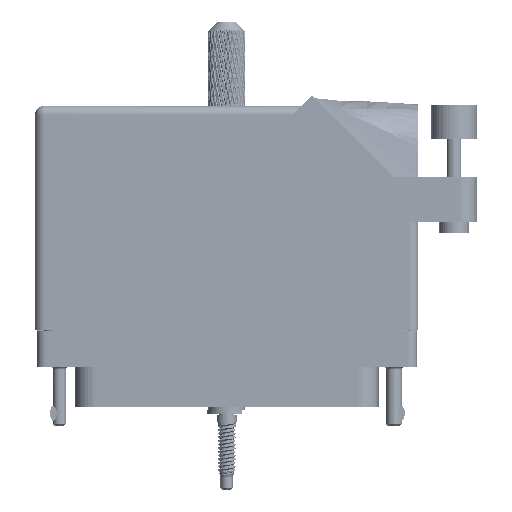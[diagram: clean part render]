
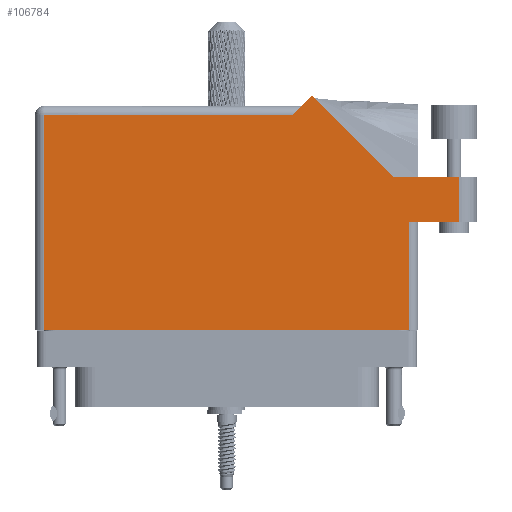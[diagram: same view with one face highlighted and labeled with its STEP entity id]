
A CAD part, front view. The second image highlights one B-rep face of the part: STEP entity #106784.
In plain terms, the highlighted face is planar.
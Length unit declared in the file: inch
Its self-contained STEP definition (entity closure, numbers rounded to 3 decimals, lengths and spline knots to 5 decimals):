
#1257 = CARTESIAN_POINT ( 'NONE',  ( 1.14042, 0.944, 0.455 ) ) ;
#1765 = ORIENTED_EDGE ( 'NONE', *, *, #94128, .T. ) ;
#3207 = ORIENTED_EDGE ( 'NONE', *, *, #35768, .T. ) ;
#3208 = ORIENTED_EDGE ( 'NONE', *, *, #44661, .T. ) ;
#7178 = CARTESIAN_POINT ( 'NONE',  ( -1.244, -0.1, 0.455 ) ) ;
#8013 = CARTESIAN_POINT ( 'NONE',  ( 1.244, 0.637, 0.455 ) ) ;
#8745 = ORIENTED_EDGE ( 'NONE', *, *, #76521, .T. ) ;
#10144 = VECTOR ( 'NONE', #37858, 39.37008 ) ;
#10283 = VERTEX_POINT ( 'NONE', #1257 ) ;
#11735 = EDGE_CURVE ( 'NONE', #63061, #35905, #89748, .T. ) ;
#12236 = DIRECTION ( 'NONE',  ( -0.707, -0.707, 0. ) ) ;
#13209 = LINE ( 'NONE', #78393, #10144 ) ;
#14014 = LINE ( 'NONE', #91039, #70665 ) ;
#14798 = DIRECTION ( 'NONE',  ( 0., -1., 0. ) ) ;
#16679 = PLANE ( 'NONE',  #77204 ) ;
#19233 = EDGE_CURVE ( 'NONE', #10283, #108725, #124353, .T. ) ;
#20253 = ORIENTED_EDGE ( 'NONE', *, *, #19233, .T. ) ;
#20635 = EDGE_CURVE ( 'NONE', #93317, #43607, #14014, .T. ) ;
#20872 = CARTESIAN_POINT ( 'NONE',  ( 0.451, 1.368, 0.455 ) ) ;
#24332 = VECTOR ( 'NONE', #41796, 39.37008 ) ;
#27872 = DIRECTION ( 'NONE',  ( -0.707, 0.707, 0. ) ) ;
#28111 = DIRECTION ( 'NONE',  ( 0., 1., 0. ) ) ;
#29269 = VERTEX_POINT ( 'NONE', #72807 ) ;
#34033 = EDGE_CURVE ( 'NONE', #51294, #62153, #13209, .T. ) ;
#35768 = EDGE_CURVE ( 'NONE', #35905, #29269, #126291, .T. ) ;
#35786 = VECTOR ( 'NONE', #27872, 39.37008 ) ;
#35905 = VERTEX_POINT ( 'NONE', #48986 ) ;
#37858 = DIRECTION ( 'NONE',  ( 0., 1., 0. ) ) ;
#37900 = ORIENTED_EDGE ( 'NONE', *, *, #34033, .T. ) ;
#41796 = DIRECTION ( 'NONE',  ( -1., 0., 0. ) ) ;
#42201 = CARTESIAN_POINT ( 'NONE',  ( 0.513, 1.43, 0.455 ) ) ;
#43607 = VERTEX_POINT ( 'NONE', #116668 ) ;
#44074 = LINE ( 'NONE', #44328, #50199 ) ;
#44328 = CARTESIAN_POINT ( 'NONE',  ( -1.244, -0.1, 0.455 ) ) ;
#44661 = EDGE_CURVE ( 'NONE', #29269, #51294, #51727, .T. ) ;
#45585 = VECTOR ( 'NONE', #108563, 39.37008 ) ;
#48986 = CARTESIAN_POINT ( 'NONE',  ( 1.244, -0.1, 0.455 ) ) ;
#50199 = VECTOR ( 'NONE', #14798, 39.37008 ) ;
#51294 = VERTEX_POINT ( 'NONE', #104453 ) ;
#51727 = LINE ( 'NONE', #88930, #45585 ) ;
#51781 = LINE ( 'NONE', #91331, #24332 ) ;
#55165 = DIRECTION ( 'NONE',  ( 0., 0., -1. ) ) ;
#58164 = CARTESIAN_POINT ( 'NONE',  ( -1.306, -0.1, 0.455 ) ) ;
#60537 = ORIENTED_EDGE ( 'NONE', *, *, #11735, .T. ) ;
#62153 = VERTEX_POINT ( 'NONE', #99463 ) ;
#63061 = VERTEX_POINT ( 'NONE', #7178 ) ;
#64982 = CARTESIAN_POINT ( 'NONE',  ( -1.306, 1.43, 0.455 ) ) ;
#70344 = EDGE_LOOP ( 'NONE', ( #3208, #37900, #97651, #20253, #8745, #115502, #1765, #60537, #3207 ) ) ;
#70665 = VECTOR ( 'NONE', #72160, 39.37008 ) ;
#72160 = DIRECTION ( 'NONE',  ( -1., 0., 0. ) ) ;
#72807 = CARTESIAN_POINT ( 'NONE',  ( 1.244, 0.637, 0.455 ) ) ;
#76521 = EDGE_CURVE ( 'NONE', #108725, #93317, #123622, .T. ) ;
#77204 = AXIS2_PLACEMENT_3D ( 'NONE', #64982, #55165, #85155 ) ;
#78393 = CARTESIAN_POINT ( 'NONE',  ( 1.581, 0.944, 0.455 ) ) ;
#79071 = VECTOR ( 'NONE', #87724, 39.37008 ) ;
#83077 = CARTESIAN_POINT ( 'NONE',  ( 1.14042, 0.944, 0.455 ) ) ;
#85155 = DIRECTION ( 'NONE',  ( -1., 0., 0. ) ) ;
#87724 = DIRECTION ( 'NONE',  ( 1., 0., 0. ) ) ;
#88590 = CARTESIAN_POINT ( 'NONE',  ( 0.58371, 1.50071, 0.455 ) ) ;
#88930 = CARTESIAN_POINT ( 'NONE',  ( 1.306, 0.637, 0.455 ) ) ;
#89748 = LINE ( 'NONE', #58164, #79071 ) ;
#91039 = CARTESIAN_POINT ( 'NONE',  ( -1.306, 1.368, 0.455 ) ) ;
#91331 = CARTESIAN_POINT ( 'NONE',  ( 1.706, 0.944, 0.455 ) ) ;
#93317 = VERTEX_POINT ( 'NONE', #20872 ) ;
#93380 = EDGE_CURVE ( 'NONE', #62153, #10283, #51781, .T. ) ;
#94128 = EDGE_CURVE ( 'NONE', #43607, #63061, #44074, .T. ) ;
#97651 = ORIENTED_EDGE ( 'NONE', *, *, #93380, .T. ) ;
#99463 = CARTESIAN_POINT ( 'NONE',  ( 1.581, 0.944, 0.455 ) ) ;
#103141 = FACE_OUTER_BOUND ( 'NONE', #70344, .T. ) ;
#104453 = CARTESIAN_POINT ( 'NONE',  ( 1.581, 0.637, 0.455 ) ) ;
#106322 = VECTOR ( 'NONE', #28111, 39.37008 ) ;
#106784 = ADVANCED_FACE ( 'NONE', ( #103141 ), #16679, .F. ) ;
#108563 = DIRECTION ( 'NONE',  ( 1., 0., 0. ) ) ;
#108725 = VERTEX_POINT ( 'NONE', #88590 ) ;
#115502 = ORIENTED_EDGE ( 'NONE', *, *, #20635, .T. ) ;
#116668 = CARTESIAN_POINT ( 'NONE',  ( -1.244, 1.368, 0.455 ) ) ;
#123622 = LINE ( 'NONE', #42201, #125115 ) ;
#124353 = LINE ( 'NONE', #83077, #35786 ) ;
#125115 = VECTOR ( 'NONE', #12236, 39.37008 ) ;
#126291 = LINE ( 'NONE', #8013, #106322 ) ;
